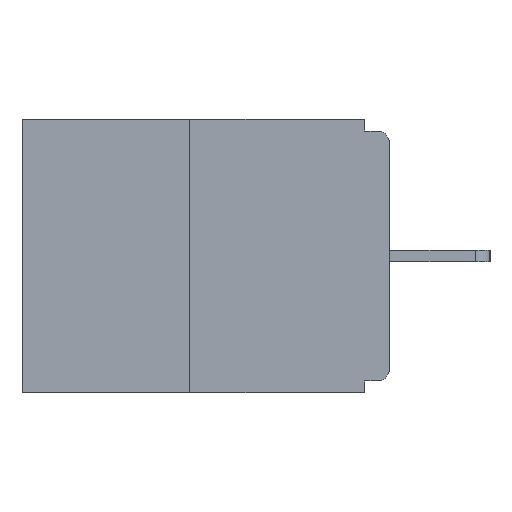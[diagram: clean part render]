
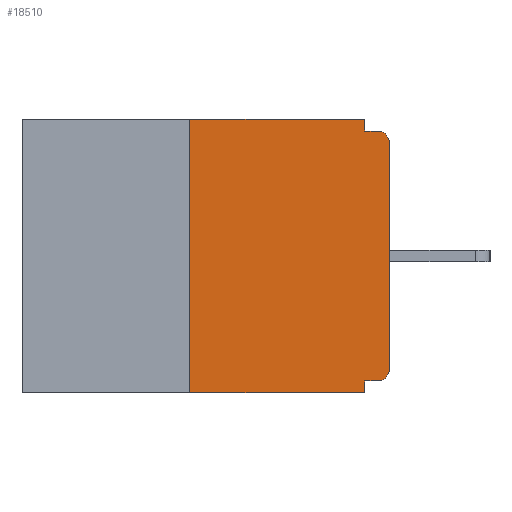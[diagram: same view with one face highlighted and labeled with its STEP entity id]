
A CAD part, left-side view. The second image highlights one B-rep face of the part: STEP entity #18510.
In plain terms, the highlighted planar face has unit normal (-1, 0, 0).
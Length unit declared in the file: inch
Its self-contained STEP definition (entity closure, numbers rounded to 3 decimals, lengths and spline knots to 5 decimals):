
#33 = DIRECTION ( 'NONE',  ( 0., 1., 0. ) ) ;
#203 = CARTESIAN_POINT ( 'NONE',  ( 0., 0.031, -0.328 ) ) ;
#319 = VECTOR ( 'NONE', #15919, 39.37008 ) ;
#368 = CARTESIAN_POINT ( 'NONE',  ( 0., 0.015, -0.328 ) ) ;
#452 = CARTESIAN_POINT ( 'NONE',  ( 0., 0.031, -0.343 ) ) ;
#657 = DIRECTION ( 'NONE',  ( 0., 0., -1. ) ) ;
#1396 = CARTESIAN_POINT ( 'NONE',  ( 0., 0.46, 0. ) ) ;
#1473 = CARTESIAN_POINT ( 'NONE',  ( 0., 0.25, 0. ) ) ;
#1513 = EDGE_CURVE ( 'NONE', #7247, #17559, #22457, .T. ) ;
#1692 = DIRECTION ( 'NONE',  ( 1., 0., 0. ) ) ;
#1882 = FACE_OUTER_BOUND ( 'NONE', #3687, .T. ) ;
#2229 = EDGE_CURVE ( 'NONE', #15646, #7247, #5149, .T. ) ;
#2273 = LINE ( 'NONE', #13337, #2578 ) ;
#2578 = VECTOR ( 'NONE', #17771, 39.37008 ) ;
#3004 = EDGE_CURVE ( 'NONE', #17559, #24184, #20564, .T. ) ;
#3300 = CARTESIAN_POINT ( 'NONE',  ( 0., 0., -0.015 ) ) ;
#3401 = DIRECTION ( 'NONE',  ( -1., 0., 0. ) ) ;
#3415 = ORIENTED_EDGE ( 'NONE', *, *, #27067, .T. ) ;
#3687 = EDGE_LOOP ( 'NONE', ( #23092, #23821, #3415, #12151, #8137, #16139, #23756, #13233, #5282, #9658 ) ) ;
#3795 = DIRECTION ( 'NONE',  ( 0., 0., -1. ) ) ;
#3808 = VECTOR ( 'NONE', #33, 39.37008 ) ;
#3830 = VECTOR ( 'NONE', #5564, 39.37008 ) ;
#4570 = VECTOR ( 'NONE', #21652, 39.37008 ) ;
#5149 = LINE ( 'NONE', #22438, #3830 ) ;
#5282 = ORIENTED_EDGE ( 'NONE', *, *, #3004, .F. ) ;
#5564 = DIRECTION ( 'NONE',  ( 0., -1., 0. ) ) ;
#5665 = CARTESIAN_POINT ( 'NONE',  ( 0., 0.031, 0. ) ) ;
#5819 = EDGE_CURVE ( 'NONE', #20982, #13542, #13162, .T. ) ;
#5898 = CARTESIAN_POINT ( 'NONE',  ( 0., 0., 0. ) ) ;
#7137 = AXIS2_PLACEMENT_3D ( 'NONE', #1396, #1692, #3795 ) ;
#7247 = VERTEX_POINT ( 'NONE', #14196 ) ;
#8137 = ORIENTED_EDGE ( 'NONE', *, *, #25313, .F. ) ;
#8388 = VERTEX_POINT ( 'NONE', #452 ) ;
#8483 = CARTESIAN_POINT ( 'NONE',  ( 0., 0.46, -0.343 ) ) ;
#8521 = LINE ( 'NONE', #5898, #11496 ) ;
#8879 = VECTOR ( 'NONE', #26219, 39.37008 ) ;
#9186 = DIRECTION ( 'NONE',  ( -1., 0., 0. ) ) ;
#9328 = CARTESIAN_POINT ( 'NONE',  ( 0., 0.015, -0.015 ) ) ;
#9658 = ORIENTED_EDGE ( 'NONE', *, *, #1513, .F. ) ;
#9871 = DIRECTION ( 'NONE',  ( 0., 0., -1. ) ) ;
#10243 = LINE ( 'NONE', #8483, #4570 ) ;
#10795 = CARTESIAN_POINT ( 'NONE',  ( 0., 0., -0.328 ) ) ;
#10803 = LINE ( 'NONE', #10795, #3808 ) ;
#11496 = VECTOR ( 'NONE', #18439, 39.37008 ) ;
#11660 = EDGE_CURVE ( 'NONE', #22143, #8388, #2273, .T. ) ;
#12151 = ORIENTED_EDGE ( 'NONE', *, *, #11660, .F. ) ;
#13162 = CIRCLE ( 'NONE', #17417, 0.015 ) ;
#13233 = ORIENTED_EDGE ( 'NONE', *, *, #19602, .T. ) ;
#13337 = CARTESIAN_POINT ( 'NONE',  ( 0., 0.031, -0.343 ) ) ;
#13542 = VERTEX_POINT ( 'NONE', #17174 ) ;
#13933 = DIRECTION ( 'NONE',  ( 0., 0., -1. ) ) ;
#14196 = CARTESIAN_POINT ( 'NONE',  ( 0., 0.031, 0. ) ) ;
#14260 = CARTESIAN_POINT ( 'NONE',  ( 0., 0.031, -0.015 ) ) ;
#15646 = VERTEX_POINT ( 'NONE', #1473 ) ;
#15919 = DIRECTION ( 'NONE',  ( 0., -1., 0. ) ) ;
#16101 = CARTESIAN_POINT ( 'NONE',  ( 0., 0.015, -0.313 ) ) ;
#16139 = ORIENTED_EDGE ( 'NONE', *, *, #5819, .T. ) ;
#16534 = PLANE ( 'NONE',  #7137 ) ;
#16863 = VERTEX_POINT ( 'NONE', #20428 ) ;
#17174 = CARTESIAN_POINT ( 'NONE',  ( 0., 0., -0.313 ) ) ;
#17417 = AXIS2_PLACEMENT_3D ( 'NONE', #16101, #3401, #9871 ) ;
#17559 = VERTEX_POINT ( 'NONE', #14260 ) ;
#17771 = DIRECTION ( 'NONE',  ( 0., 0., -1. ) ) ;
#18068 = EDGE_CURVE ( 'NONE', #16863, #15646, #25422, .T. ) ;
#18439 = DIRECTION ( 'NONE',  ( 0., 0., 1. ) ) ;
#18510 = ADVANCED_FACE ( 'NONE', ( #1882 ), #16534, .F. ) ;
#19602 = EDGE_CURVE ( 'NONE', #21190, #24184, #19826, .T. ) ;
#19826 = CIRCLE ( 'NONE', #27410, 0.015 ) ;
#19952 = CARTESIAN_POINT ( 'NONE',  ( 0., 0.25, 0. ) ) ;
#20428 = CARTESIAN_POINT ( 'NONE',  ( 0., 0.25, -0.343 ) ) ;
#20564 = LINE ( 'NONE', #3300, #319 ) ;
#20982 = VERTEX_POINT ( 'NONE', #368 ) ;
#21190 = VERTEX_POINT ( 'NONE', #26087 ) ;
#21652 = DIRECTION ( 'NONE',  ( 0., -1., 0. ) ) ;
#21791 = VECTOR ( 'NONE', #13933, 39.37008 ) ;
#22143 = VERTEX_POINT ( 'NONE', #203 ) ;
#22270 = CARTESIAN_POINT ( 'NONE',  ( 0., 0.015, -0.03 ) ) ;
#22438 = CARTESIAN_POINT ( 'NONE',  ( 0., 0.46, 0. ) ) ;
#22457 = LINE ( 'NONE', #5665, #21791 ) ;
#23092 = ORIENTED_EDGE ( 'NONE', *, *, #2229, .F. ) ;
#23756 = ORIENTED_EDGE ( 'NONE', *, *, #24369, .T. ) ;
#23821 = ORIENTED_EDGE ( 'NONE', *, *, #18068, .F. ) ;
#24184 = VERTEX_POINT ( 'NONE', #9328 ) ;
#24369 = EDGE_CURVE ( 'NONE', #13542, #21190, #8521, .T. ) ;
#25313 = EDGE_CURVE ( 'NONE', #20982, #22143, #10803, .T. ) ;
#25422 = LINE ( 'NONE', #19952, #8879 ) ;
#26087 = CARTESIAN_POINT ( 'NONE',  ( 0., 0., -0.03 ) ) ;
#26219 = DIRECTION ( 'NONE',  ( 0., 0., 1. ) ) ;
#27067 = EDGE_CURVE ( 'NONE', #16863, #8388, #10243, .T. ) ;
#27410 = AXIS2_PLACEMENT_3D ( 'NONE', #22270, #9186, #657 ) ;
